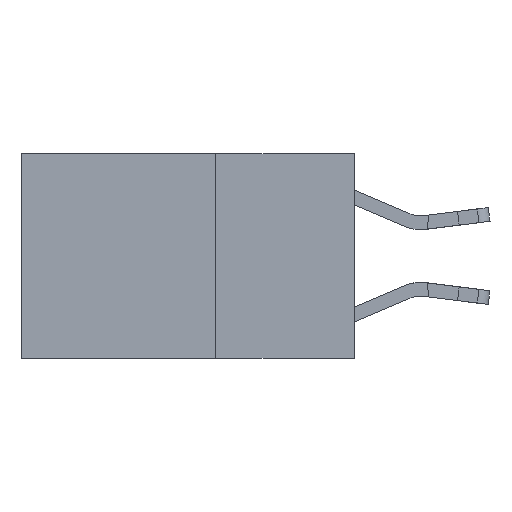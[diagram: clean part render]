
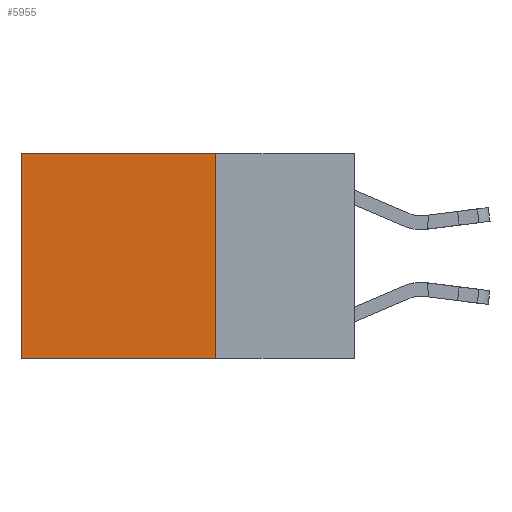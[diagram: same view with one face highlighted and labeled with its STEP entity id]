
A CAD part, left-side view. The second image highlights one B-rep face of the part: STEP entity #5955.
In plain terms, the highlighted planar face has unit normal (-1, 0, 0).
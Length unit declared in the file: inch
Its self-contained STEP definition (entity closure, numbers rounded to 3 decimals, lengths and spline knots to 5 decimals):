
#225 = DIRECTION ( 'NONE',  ( 0., 0., -1. ) ) ;
#506 = EDGE_CURVE ( 'NONE', #9779, #13473, #13921, .T. ) ;
#624 = VECTOR ( 'NONE', #225, 39.37008 ) ;
#1292 = DIRECTION ( 'NONE',  ( 0., 1., 0. ) ) ;
#1313 = LINE ( 'NONE', #13957, #3584 ) ;
#2042 = ORIENTED_EDGE ( 'NONE', *, *, #2397, .T. ) ;
#2397 = EDGE_CURVE ( 'NONE', #12712, #13473, #3860, .T. ) ;
#2429 = CARTESIAN_POINT ( 'NONE',  ( 0.2625, 0.25, 0. ) ) ;
#2522 = ORIENTED_EDGE ( 'NONE', *, *, #7186, .T. ) ;
#2848 = DIRECTION ( 'NONE',  ( 0., 0., -1. ) ) ;
#3092 = CARTESIAN_POINT ( 'NONE',  ( 0.2625, 0.6, -0.37 ) ) ;
#3534 = VECTOR ( 'NONE', #1292, 39.37008 ) ;
#3584 = VECTOR ( 'NONE', #11542, 39.37008 ) ;
#3860 = LINE ( 'NONE', #11256, #624 ) ;
#4026 = VERTEX_POINT ( 'NONE', #11677 ) ;
#4898 = PLANE ( 'NONE',  #13674 ) ;
#4905 = FACE_OUTER_BOUND ( 'NONE', #12804, .T. ) ;
#5235 = ORIENTED_EDGE ( 'NONE', *, *, #506, .F. ) ;
#5390 = LINE ( 'NONE', #2429, #11731 ) ;
#5955 = ADVANCED_FACE ( 'NONE', ( #4905 ), #4898, .F. ) ;
#5996 = CARTESIAN_POINT ( 'NONE',  ( 0.2625, 0.25, 0. ) ) ;
#6140 = DIRECTION ( 'NONE',  ( 1., 0., 0. ) ) ;
#7186 = EDGE_CURVE ( 'NONE', #4026, #12712, #1313, .T. ) ;
#9051 = CARTESIAN_POINT ( 'NONE',  ( 0.2625, 0.6, 0. ) ) ;
#9779 = VERTEX_POINT ( 'NONE', #10121 ) ;
#10121 = CARTESIAN_POINT ( 'NONE',  ( 0.2625, 0.25, -0.37 ) ) ;
#10797 = EDGE_CURVE ( 'NONE', #4026, #9779, #5390, .T. ) ;
#11256 = CARTESIAN_POINT ( 'NONE',  ( 0.2625, 0.6, 0. ) ) ;
#11542 = DIRECTION ( 'NONE',  ( 0., 1., 0. ) ) ;
#11677 = CARTESIAN_POINT ( 'NONE',  ( 0.2625, 0.25, 0. ) ) ;
#11731 = VECTOR ( 'NONE', #2848, 39.37008 ) ;
#12712 = VERTEX_POINT ( 'NONE', #9051 ) ;
#12804 = EDGE_LOOP ( 'NONE', ( #2042, #5235, #13364, #2522 ) ) ;
#13285 = CARTESIAN_POINT ( 'NONE',  ( 0.2625, 0.25, -0.37 ) ) ;
#13364 = ORIENTED_EDGE ( 'NONE', *, *, #10797, .F. ) ;
#13473 = VERTEX_POINT ( 'NONE', #3092 ) ;
#13674 = AXIS2_PLACEMENT_3D ( 'NONE', #5996, #6140, #14705 ) ;
#13921 = LINE ( 'NONE', #13285, #3534 ) ;
#13957 = CARTESIAN_POINT ( 'NONE',  ( 0.2625, 0.25, 0. ) ) ;
#14705 = DIRECTION ( 'NONE',  ( 0., 0., -1. ) ) ;
